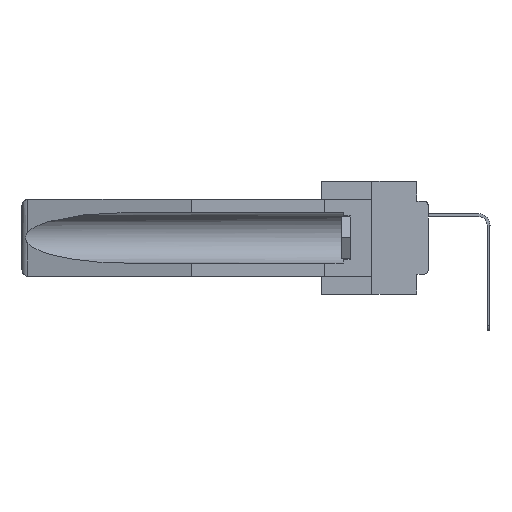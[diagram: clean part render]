
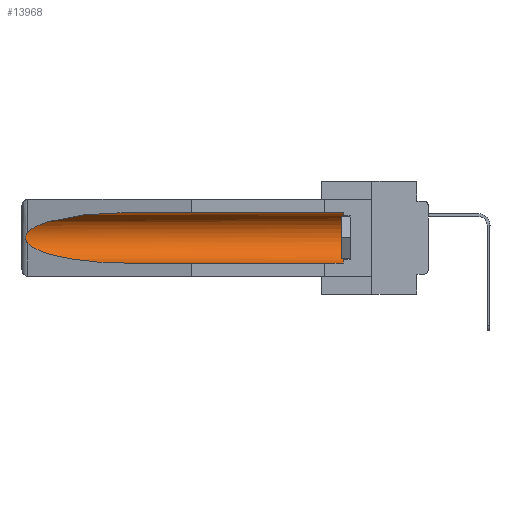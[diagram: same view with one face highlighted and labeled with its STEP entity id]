
A CAD part, left-side view. The second image highlights one B-rep face of the part: STEP entity #13968.
In plain terms, the highlighted cylindrical face has radius 2.857 mm (diameter 5.715 mm), a partial arc.
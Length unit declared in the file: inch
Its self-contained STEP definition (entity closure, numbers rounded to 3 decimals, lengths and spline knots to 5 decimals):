
#90 = CARTESIAN_POINT ( 'NONE',  ( 0.2673, 1.53269, -0.17917 ) ) ;
#1364 =( BOUNDED_CURVE ( )  B_SPLINE_CURVE ( 3, ( #15863, #2622, #12904, #31435 ),
 .UNSPECIFIED., .F., .F. ) 
 B_SPLINE_CURVE_WITH_KNOTS ( ( 4, 4 ),
 ( 4.71239, 6.08839 ),
 .UNSPECIFIED. ) 
 CURVE ( )  GEOMETRIC_REPRESENTATION_ITEM ( )  RATIONAL_B_SPLINE_CURVE ( ( 1., 0.848, 0.848, 1. ) ) 
 REPRESENTATION_ITEM ( '' )  );
#1478 = VECTOR ( 'NONE', #19630, 39.37008 ) ;
#1503 = VERTEX_POINT ( 'NONE', #12854 ) ;
#2009 = AXIS2_PLACEMENT_3D ( 'NONE', #20898, #2047, #4894 ) ;
#2047 = DIRECTION ( 'NONE',  ( 0., 1., 0. ) ) ;
#2404 = EDGE_CURVE ( 'NONE', #9646, #1503, #9271, .T. ) ;
#2622 = CARTESIAN_POINT ( 'NONE',  ( 0.21114, 1.30732, -0.059 ) ) ;
#2730 = CARTESIAN_POINT ( 'NONE',  ( 0.26655, 1.53094, -0.18657 ) ) ;
#2836 = FACE_OUTER_BOUND ( 'NONE', #25580, .T. ) ;
#3151 = ORIENTED_EDGE ( 'NONE', *, *, #9721, .T. ) ;
#4071 = EDGE_CURVE ( 'NONE', #1503, #32679, #11721, .T. ) ;
#4362 = AXIS2_PLACEMENT_3D ( 'NONE', #32957, #14856, #14757 ) ;
#4714 = EDGE_CURVE ( 'NONE', #34032, #28978, #4739, .T. ) ;
#4739 = B_SPLINE_CURVE_WITH_KNOTS ( 'NONE', 3,
 ( #15614, #20905, #18350, #31648, #20797, #7546, #90, #2730, #7663, #20687 ),
 .UNSPECIFIED., .F., .F.,
 ( 4, 2, 2, 2, 4 ),
 ( 0., 0.00029, 0.00058, 0.00087, 0.00117 ),
 .UNSPECIFIED. ) ;
#4894 = DIRECTION ( 'NONE',  ( 0., 0., 1. ) ) ;
#6518 = CARTESIAN_POINT ( 'NONE',  ( 0.155, 1.07973, -0.284 ) ) ;
#6852 = CARTESIAN_POINT ( 'NONE',  ( 0.21114, 1.30732, -0.284 ) ) ;
#7091 = ORIENTED_EDGE ( 'NONE', *, *, #2404, .T. ) ;
#7264 = CARTESIAN_POINT ( 'NONE',  ( 0.155, 1.07973, -0.284 ) ) ;
#7546 = CARTESIAN_POINT ( 'NONE',  ( 0.2675, 1.53308, -0.17534 ) ) ;
#7649 = VERTEX_POINT ( 'NONE', #7264 ) ;
#7663 = CARTESIAN_POINT ( 'NONE',  ( 0.26597, 1.5296, -0.19026 ) ) ;
#9063 = CARTESIAN_POINT ( 'NONE',  ( 0.26537, 1.52718, -0.19328 ) ) ;
#9271 = CIRCLE ( 'NONE', #4362, 0.1125 ) ;
#9646 = VERTEX_POINT ( 'NONE', #24291 ) ;
#9721 = EDGE_CURVE ( 'NONE', #28978, #7649, #26704, .T. ) ;
#10051 = DIRECTION ( 'NONE',  ( 0., 1., 0. ) ) ;
#10302 = CYLINDRICAL_SURFACE ( 'NONE', #2009, 0.1125 ) ;
#11721 = LINE ( 'NONE', #28443, #32299 ) ;
#12854 = CARTESIAN_POINT ( 'NONE',  ( 0.155, 0.126, -0.059 ) ) ;
#12904 = CARTESIAN_POINT ( 'NONE',  ( 0.25451, 1.48313, -0.09465 ) ) ;
#13968 = ADVANCED_FACE ( 'NONE', ( #2836 ), #10302, .F. ) ;
#14757 = DIRECTION ( 'NONE',  ( 0., 0., 1. ) ) ;
#14856 = DIRECTION ( 'NONE',  ( 0., -1., 0. ) ) ;
#15614 = CARTESIAN_POINT ( 'NONE',  ( 0.26537, 1.52718, -0.14972 ) ) ;
#15863 = CARTESIAN_POINT ( 'NONE',  ( 0.155, 1.07973, -0.059 ) ) ;
#16054 = CARTESIAN_POINT ( 'NONE',  ( 0.155, 1.07973, -0.059 ) ) ;
#17160 = ORIENTED_EDGE ( 'NONE', *, *, #4071, .T. ) ;
#18350 = CARTESIAN_POINT ( 'NONE',  ( 0.26654, 1.53092, -0.15636 ) ) ;
#19630 = DIRECTION ( 'NONE',  ( 0., 1., 0. ) ) ;
#20687 = CARTESIAN_POINT ( 'NONE',  ( 0.26537, 1.52718, -0.19328 ) ) ;
#20797 = CARTESIAN_POINT ( 'NONE',  ( 0.2675, 1.53308, -0.16763 ) ) ;
#20898 = CARTESIAN_POINT ( 'NONE',  ( 0.155, -0.30754, -0.1715 ) ) ;
#20905 = CARTESIAN_POINT ( 'NONE',  ( 0.26597, 1.52961, -0.15275 ) ) ;
#22987 = EDGE_CURVE ( 'NONE', #9646, #7649, #24141, .T. ) ;
#23454 = ORIENTED_EDGE ( 'NONE', *, *, #4714, .T. ) ;
#24141 = LINE ( 'NONE', #24711, #1478 ) ;
#24291 = CARTESIAN_POINT ( 'NONE',  ( 0.155, 0.126, -0.284 ) ) ;
#24711 = CARTESIAN_POINT ( 'NONE',  ( 0.155, -0.30754, -0.284 ) ) ;
#25055 = EDGE_CURVE ( 'NONE', #32679, #34032, #1364, .T. ) ;
#25580 = EDGE_LOOP ( 'NONE', ( #31403, #23454, #3151, #31982, #7091, #17160 ) ) ;
#26704 =( BOUNDED_CURVE ( )  B_SPLINE_CURVE ( 3, ( #9063, #30485, #6852, #6518 ),
 .UNSPECIFIED., .F., .T. ) 
 B_SPLINE_CURVE_WITH_KNOTS ( ( 4, 4 ),
 ( 0.1948, 1.5708 ),
 .UNSPECIFIED. ) 
 CURVE ( )  GEOMETRIC_REPRESENTATION_ITEM ( )  RATIONAL_B_SPLINE_CURVE ( ( 1., 0.848, 0.848, 1. ) ) 
 REPRESENTATION_ITEM ( '' )  );
#26926 = CARTESIAN_POINT ( 'NONE',  ( 0.26537, 1.52718, -0.14972 ) ) ;
#27343 = CARTESIAN_POINT ( 'NONE',  ( 0.26537, 1.52718, -0.19328 ) ) ;
#28443 = CARTESIAN_POINT ( 'NONE',  ( 0.155, -0.30754, -0.059 ) ) ;
#28978 = VERTEX_POINT ( 'NONE', #27343 ) ;
#30485 = CARTESIAN_POINT ( 'NONE',  ( 0.25451, 1.48313, -0.24835 ) ) ;
#31403 = ORIENTED_EDGE ( 'NONE', *, *, #25055, .T. ) ;
#31435 = CARTESIAN_POINT ( 'NONE',  ( 0.26537, 1.52718, -0.14972 ) ) ;
#31648 = CARTESIAN_POINT ( 'NONE',  ( 0.2673, 1.5327, -0.16383 ) ) ;
#31982 = ORIENTED_EDGE ( 'NONE', *, *, #22987, .F. ) ;
#32299 = VECTOR ( 'NONE', #10051, 39.37008 ) ;
#32679 = VERTEX_POINT ( 'NONE', #16054 ) ;
#32957 = CARTESIAN_POINT ( 'NONE',  ( 0.155, 0.126, -0.1715 ) ) ;
#34032 = VERTEX_POINT ( 'NONE', #26926 ) ;
